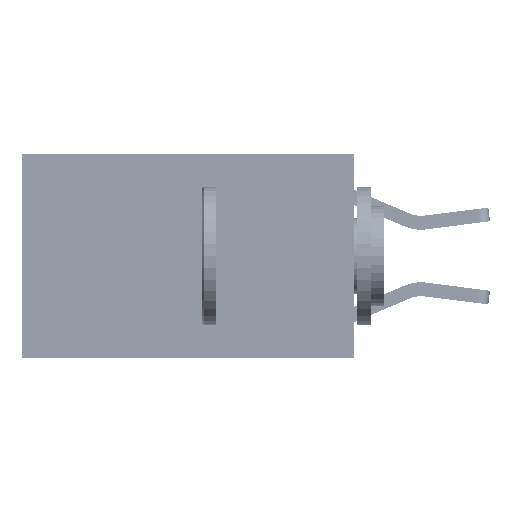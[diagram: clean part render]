
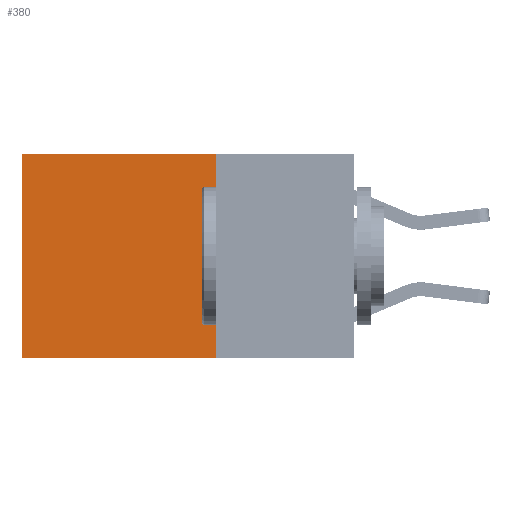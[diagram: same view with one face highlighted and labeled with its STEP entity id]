
A CAD part, left-side view. The second image highlights one B-rep face of the part: STEP entity #380.
In plain terms, the highlighted planar face has unit normal (-1, 0, 0).
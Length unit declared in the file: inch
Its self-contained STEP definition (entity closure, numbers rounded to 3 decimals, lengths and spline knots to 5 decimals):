
#380 = ADVANCED_FACE ( 'NONE', ( #10969 ), #803, .F. ) ;
#792 = DIRECTION ( 'NONE',  ( 0., 0., -1. ) ) ;
#803 = PLANE ( 'NONE',  #27941 ) ;
#1899 = DIRECTION ( 'NONE',  ( 0., 1., 0. ) ) ;
#4164 = VECTOR ( 'NONE', #1899, 39.37008 ) ;
#4567 = ORIENTED_EDGE ( 'NONE', *, *, #18484, .T. ) ;
#5338 = VERTEX_POINT ( 'NONE', #9232 ) ;
#5801 = CARTESIAN_POINT ( 'NONE',  ( 0.2625, 0.25, 0. ) ) ;
#9232 = CARTESIAN_POINT ( 'NONE',  ( 0.2625, 0.25, -0.37 ) ) ;
#10969 = FACE_OUTER_BOUND ( 'NONE', #12110, .T. ) ;
#11998 = VECTOR ( 'NONE', #27059, 39.37008 ) ;
#12110 = EDGE_LOOP ( 'NONE', ( #18368, #27201, #16511, #4567 ) ) ;
#13220 = VECTOR ( 'NONE', #792, 39.37008 ) ;
#13734 = VERTEX_POINT ( 'NONE', #32312 ) ;
#16511 = ORIENTED_EDGE ( 'NONE', *, *, #26181, .F. ) ;
#16877 = LINE ( 'NONE', #29731, #11998 ) ;
#18368 = ORIENTED_EDGE ( 'NONE', *, *, #21637, .T. ) ;
#18484 = EDGE_CURVE ( 'NONE', #26313, #13734, #23740, .T. ) ;
#18501 = DIRECTION ( 'NONE',  ( 0., 0., -1. ) ) ;
#18824 = DIRECTION ( 'NONE',  ( 1., 0., 0. ) ) ;
#19104 = LINE ( 'NONE', #29297, #4164 ) ;
#19196 = VECTOR ( 'NONE', #29415, 39.37008 ) ;
#21637 = EDGE_CURVE ( 'NONE', #13734, #28484, #16877, .T. ) ;
#23740 = LINE ( 'NONE', #26578, #19196 ) ;
#24817 = CARTESIAN_POINT ( 'NONE',  ( 0.2625, 0.25, 0. ) ) ;
#26181 = EDGE_CURVE ( 'NONE', #26313, #5338, #31184, .T. ) ;
#26313 = VERTEX_POINT ( 'NONE', #24817 ) ;
#26578 = CARTESIAN_POINT ( 'NONE',  ( 0.2625, 0.25, 0. ) ) ;
#26880 = EDGE_CURVE ( 'NONE', #5338, #28484, #19104, .T. ) ;
#27059 = DIRECTION ( 'NONE',  ( 0., 0., -1. ) ) ;
#27201 = ORIENTED_EDGE ( 'NONE', *, *, #26880, .F. ) ;
#27941 = AXIS2_PLACEMENT_3D ( 'NONE', #5801, #18824, #18501 ) ;
#28484 = VERTEX_POINT ( 'NONE', #32469 ) ;
#28518 = CARTESIAN_POINT ( 'NONE',  ( 0.2625, 0.25, 0. ) ) ;
#29297 = CARTESIAN_POINT ( 'NONE',  ( 0.2625, 0.25, -0.37 ) ) ;
#29415 = DIRECTION ( 'NONE',  ( 0., 1., 0. ) ) ;
#29731 = CARTESIAN_POINT ( 'NONE',  ( 0.2625, 0.6, 0. ) ) ;
#31184 = LINE ( 'NONE', #28518, #13220 ) ;
#32312 = CARTESIAN_POINT ( 'NONE',  ( 0.2625, 0.6, 0. ) ) ;
#32469 = CARTESIAN_POINT ( 'NONE',  ( 0.2625, 0.6, -0.37 ) ) ;
